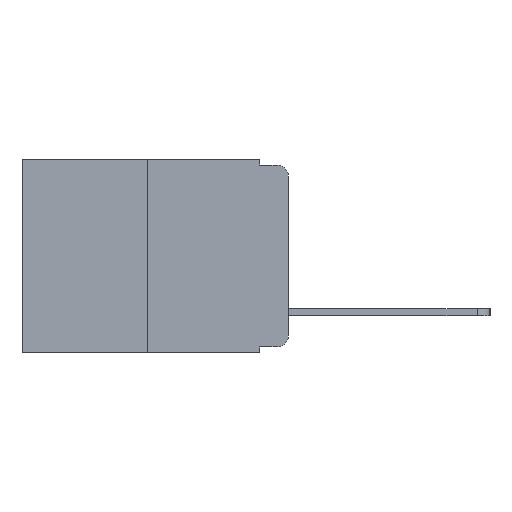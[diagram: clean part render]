
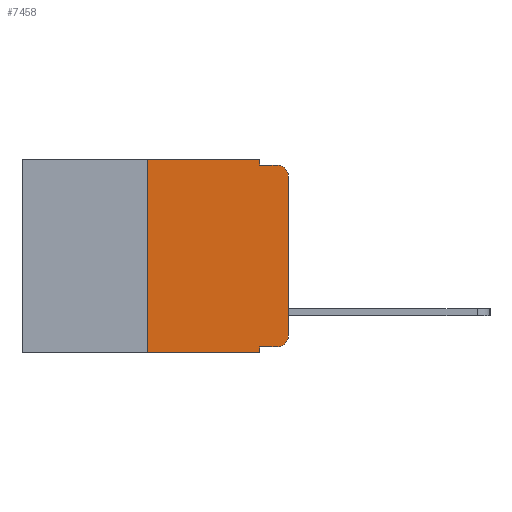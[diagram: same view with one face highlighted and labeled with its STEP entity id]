
A CAD part, left-side view. The second image highlights one B-rep face of the part: STEP entity #7458.
In plain terms, the highlighted planar face has unit normal (-1, 0, 0).
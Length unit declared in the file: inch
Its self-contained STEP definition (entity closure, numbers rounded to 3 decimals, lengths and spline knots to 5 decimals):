
#24 = CARTESIAN_POINT ( 'NONE',  ( 0., 0.02, -0.03 ) ) ;
#192 = EDGE_CURVE ( 'NONE', #5968, #9678, #9801, .T. ) ;
#218 = AXIS2_PLACEMENT_3D ( 'NONE', #1984, #6071, #12773 ) ;
#298 = AXIS2_PLACEMENT_3D ( 'NONE', #24, #7149, #1061 ) ;
#330 = CARTESIAN_POINT ( 'NONE',  ( 0., 0.051, -0.333 ) ) ;
#399 = VERTEX_POINT ( 'NONE', #12198 ) ;
#414 = EDGE_CURVE ( 'NONE', #399, #9678, #2614, .T. ) ;
#1061 = DIRECTION ( 'NONE',  ( 0., 0., -1. ) ) ;
#1160 = CARTESIAN_POINT ( 'NONE',  ( 0., 0., -0.313 ) ) ;
#1265 = ORIENTED_EDGE ( 'NONE', *, *, #9618, .T. ) ;
#1277 = ORIENTED_EDGE ( 'NONE', *, *, #5898, .T. ) ;
#1375 = LINE ( 'NONE', #4656, #11300 ) ;
#1387 = CARTESIAN_POINT ( 'NONE',  ( 0., 0.051, -0.333 ) ) ;
#1561 = ORIENTED_EDGE ( 'NONE', *, *, #7005, .T. ) ;
#1984 = CARTESIAN_POINT ( 'NONE',  ( 0., 0.473, 0. ) ) ;
#2201 = DIRECTION ( 'NONE',  ( -1., 0., 0. ) ) ;
#2387 = VECTOR ( 'NONE', #10400, 39.37008 ) ;
#2614 = LINE ( 'NONE', #12025, #7687 ) ;
#2619 = VERTEX_POINT ( 'NONE', #12733 ) ;
#2806 = CARTESIAN_POINT ( 'NONE',  ( 0., 0.25, 0. ) ) ;
#2815 = VECTOR ( 'NONE', #6353, 39.37008 ) ;
#2941 = EDGE_CURVE ( 'NONE', #399, #8173, #10040, .T. ) ;
#3976 = VECTOR ( 'NONE', #5922, 39.37008 ) ;
#4045 = CARTESIAN_POINT ( 'NONE',  ( 0., 0.02, -0.333 ) ) ;
#4180 = DIRECTION ( 'NONE',  ( 0., 0., -1. ) ) ;
#4369 = ORIENTED_EDGE ( 'NONE', *, *, #5664, .F. ) ;
#4582 = VECTOR ( 'NONE', #4180, 39.37008 ) ;
#4656 = CARTESIAN_POINT ( 'NONE',  ( 0., 0., 0. ) ) ;
#4745 = LINE ( 'NONE', #7750, #12123 ) ;
#4751 = EDGE_CURVE ( 'NONE', #8173, #12440, #11136, .T. ) ;
#4998 = ORIENTED_EDGE ( 'NONE', *, *, #4751, .F. ) ;
#5020 = EDGE_CURVE ( 'NONE', #12440, #2619, #10699, .T. ) ;
#5301 = ORIENTED_EDGE ( 'NONE', *, *, #2941, .F. ) ;
#5375 = CARTESIAN_POINT ( 'NONE',  ( 0., 0.051, 0. ) ) ;
#5443 = LINE ( 'NONE', #1387, #2387 ) ;
#5600 = ORIENTED_EDGE ( 'NONE', *, *, #414, .T. ) ;
#5639 = DIRECTION ( 'NONE',  ( 0., 0., 1. ) ) ;
#5664 = EDGE_CURVE ( 'NONE', #2619, #9769, #4745, .T. ) ;
#5898 = EDGE_CURVE ( 'NONE', #9086, #10139, #6590, .T. ) ;
#5922 = DIRECTION ( 'NONE',  ( 0., -1., 0. ) ) ;
#5968 = VERTEX_POINT ( 'NONE', #330 ) ;
#6071 = DIRECTION ( 'NONE',  ( 1., 0., 0. ) ) ;
#6353 = DIRECTION ( 'NONE',  ( 0., 0., -1. ) ) ;
#6590 = CIRCLE ( 'NONE', #7091, 0.02 ) ;
#6598 = CARTESIAN_POINT ( 'NONE',  ( 0., 0., -0.03 ) ) ;
#6757 = CARTESIAN_POINT ( 'NONE',  ( 0., 0.25, 0. ) ) ;
#7005 = EDGE_CURVE ( 'NONE', #7690, #9769, #9347, .T. ) ;
#7091 = AXIS2_PLACEMENT_3D ( 'NONE', #8282, #2201, #9244 ) ;
#7149 = DIRECTION ( 'NONE',  ( -1., 0., 0. ) ) ;
#7458 = ADVANCED_FACE ( 'NONE', ( #10642 ), #11827, .F. ) ;
#7655 = CARTESIAN_POINT ( 'NONE',  ( 0., 0.051, -0.343 ) ) ;
#7687 = VECTOR ( 'NONE', #10686, 39.37008 ) ;
#7690 = VERTEX_POINT ( 'NONE', #6598 ) ;
#7750 = CARTESIAN_POINT ( 'NONE',  ( 0., 0.051, -0.01 ) ) ;
#7779 = VECTOR ( 'NONE', #9422, 39.37008 ) ;
#8173 = VERTEX_POINT ( 'NONE', #6757 ) ;
#8282 = CARTESIAN_POINT ( 'NONE',  ( 0., 0.02, -0.313 ) ) ;
#8517 = EDGE_LOOP ( 'NONE', ( #1265, #1561, #4369, #9897, #4998, #5301, #5600, #11059, #10627, #1277 ) ) ;
#8600 = EDGE_CURVE ( 'NONE', #5968, #9086, #5443, .T. ) ;
#8824 = CARTESIAN_POINT ( 'NONE',  ( 0., 0.02, -0.01 ) ) ;
#8845 = CARTESIAN_POINT ( 'NONE',  ( 0., 0.051, 0. ) ) ;
#9086 = VERTEX_POINT ( 'NONE', #4045 ) ;
#9244 = DIRECTION ( 'NONE',  ( 0., 0., -1. ) ) ;
#9347 = CIRCLE ( 'NONE', #298, 0.02 ) ;
#9422 = DIRECTION ( 'NONE',  ( 0., 0., 1. ) ) ;
#9618 = EDGE_CURVE ( 'NONE', #10139, #7690, #1375, .T. ) ;
#9678 = VERTEX_POINT ( 'NONE', #7655 ) ;
#9769 = VERTEX_POINT ( 'NONE', #8824 ) ;
#9801 = LINE ( 'NONE', #8845, #4582 ) ;
#9897 = ORIENTED_EDGE ( 'NONE', *, *, #5020, .F. ) ;
#10040 = LINE ( 'NONE', #2806, #7779 ) ;
#10139 = VERTEX_POINT ( 'NONE', #1160 ) ;
#10219 = CARTESIAN_POINT ( 'NONE',  ( 0., 0.051, 0. ) ) ;
#10400 = DIRECTION ( 'NONE',  ( 0., -1., 0. ) ) ;
#10627 = ORIENTED_EDGE ( 'NONE', *, *, #8600, .T. ) ;
#10642 = FACE_OUTER_BOUND ( 'NONE', #8517, .T. ) ;
#10686 = DIRECTION ( 'NONE',  ( 0., -1., 0. ) ) ;
#10699 = LINE ( 'NONE', #5375, #2815 ) ;
#11059 = ORIENTED_EDGE ( 'NONE', *, *, #192, .F. ) ;
#11136 = LINE ( 'NONE', #11698, #3976 ) ;
#11300 = VECTOR ( 'NONE', #5639, 39.37008 ) ;
#11698 = CARTESIAN_POINT ( 'NONE',  ( 0., 0.473, 0. ) ) ;
#11827 = PLANE ( 'NONE',  #218 ) ;
#12025 = CARTESIAN_POINT ( 'NONE',  ( 0., 0.473, -0.343 ) ) ;
#12123 = VECTOR ( 'NONE', #12445, 39.37008 ) ;
#12198 = CARTESIAN_POINT ( 'NONE',  ( 0., 0.25, -0.343 ) ) ;
#12440 = VERTEX_POINT ( 'NONE', #10219 ) ;
#12445 = DIRECTION ( 'NONE',  ( 0., -1., 0. ) ) ;
#12733 = CARTESIAN_POINT ( 'NONE',  ( 0., 0.051, -0.01 ) ) ;
#12773 = DIRECTION ( 'NONE',  ( 0., 0., -1. ) ) ;
